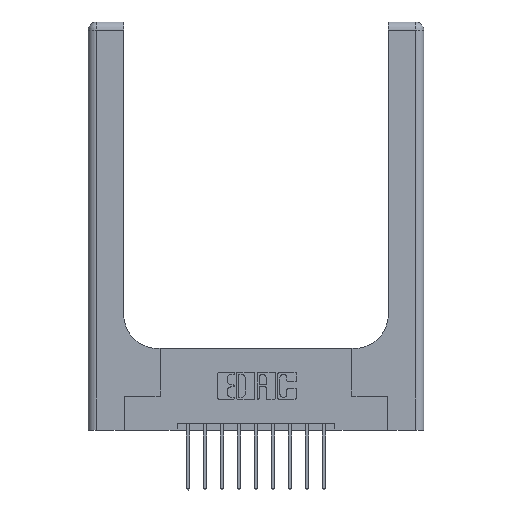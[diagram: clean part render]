
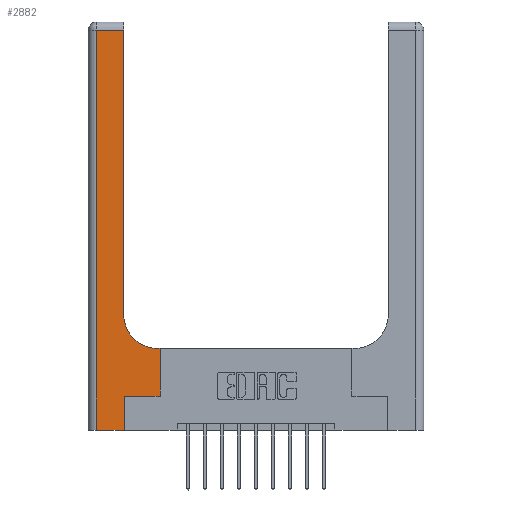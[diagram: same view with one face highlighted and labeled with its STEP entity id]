
A CAD part, top view. The second image highlights one B-rep face of the part: STEP entity #2882.
In plain terms, the highlighted planar face has unit normal (0, 0, 1).
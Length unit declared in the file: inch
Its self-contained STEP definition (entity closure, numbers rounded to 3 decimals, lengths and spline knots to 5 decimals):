
#77 = DIRECTION ( 'NONE',  ( 1., 0., 0. ) ) ;
#136 = DIRECTION ( 'NONE',  ( 0., 0., -1. ) ) ;
#170 = ORIENTED_EDGE ( 'NONE', *, *, #11150, .T. ) ;
#404 = CARTESIAN_POINT ( 'NONE',  ( 0.528, 0.6, 0.37 ) ) ;
#594 = LINE ( 'NONE', #11802, #10375 ) ;
#820 = VERTEX_POINT ( 'NONE', #9090 ) ;
#903 = LINE ( 'NONE', #4842, #3934 ) ;
#1063 = VECTOR ( 'NONE', #1886, 39.37008 ) ;
#1191 = EDGE_CURVE ( 'NONE', #10595, #3050, #9981, .T. ) ;
#1203 = CARTESIAN_POINT ( 'NONE',  ( 0., 2.94, 0.37 ) ) ;
#1225 = DIRECTION ( 'NONE',  ( 1., 0., 0. ) ) ;
#1389 = VERTEX_POINT ( 'NONE', #7661 ) ;
#1886 = DIRECTION ( 'NONE',  ( 0., 1., 0. ) ) ;
#2352 = ORIENTED_EDGE ( 'NONE', *, *, #10914, .T. ) ;
#2474 = ORIENTED_EDGE ( 'NONE', *, *, #1191, .T. ) ;
#2657 = CARTESIAN_POINT ( 'NONE',  ( 0.265, 0.25, 0.37 ) ) ;
#2847 = CARTESIAN_POINT ( 'NONE',  ( 0.528, 0.25, 0.37 ) ) ;
#2882 = ADVANCED_FACE ( 'NONE', ( #11355 ), #9747, .F. ) ;
#2932 = ORIENTED_EDGE ( 'NONE', *, *, #10328, .T. ) ;
#3050 = VERTEX_POINT ( 'NONE', #5064 ) ;
#3463 = ORIENTED_EDGE ( 'NONE', *, *, #4108, .T. ) ;
#3573 = EDGE_LOOP ( 'NONE', ( #170, #13850, #3463, #10196, #9237, #2932, #2352, #2474, #8251 ) ) ;
#3771 = DIRECTION ( 'NONE',  ( 0., -1., 0. ) ) ;
#3934 = VECTOR ( 'NONE', #13208, 39.37008 ) ;
#4108 = EDGE_CURVE ( 'NONE', #820, #1389, #4949, .T. ) ;
#4452 = LINE ( 'NONE', #10694, #8943 ) ;
#4736 = DIRECTION ( 'NONE',  ( -1., 0., 0. ) ) ;
#4842 = CARTESIAN_POINT ( 'NONE',  ( 0.265, 0.25, 0.37 ) ) ;
#4949 = LINE ( 'NONE', #8571, #5700 ) ;
#5064 = CARTESIAN_POINT ( 'NONE',  ( 0.51, 0.6, 0.37 ) ) ;
#5229 = LINE ( 'NONE', #12991, #8219 ) ;
#5380 = VERTEX_POINT ( 'NONE', #8799 ) ;
#5700 = VECTOR ( 'NONE', #3771, 39.37008 ) ;
#6095 = EDGE_CURVE ( 'NONE', #3050, #5380, #8255, .T. ) ;
#6099 = DIRECTION ( 'NONE',  ( 0., 0., -1. ) ) ;
#6612 = AXIS2_PLACEMENT_3D ( 'NONE', #13303, #136, #77 ) ;
#7354 = EDGE_CURVE ( 'NONE', #14224, #820, #14974, .T. ) ;
#7412 = VERTEX_POINT ( 'NONE', #2847 ) ;
#7661 = CARTESIAN_POINT ( 'NONE',  ( 0.06, 0., 0.37 ) ) ;
#8140 = DIRECTION ( 'NONE',  ( 0., 1., 0. ) ) ;
#8219 = VECTOR ( 'NONE', #8271, 39.37008 ) ;
#8251 = ORIENTED_EDGE ( 'NONE', *, *, #6095, .T. ) ;
#8255 = CIRCLE ( 'NONE', #6612, 0.25 ) ;
#8271 = DIRECTION ( 'NONE',  ( 0., 1., 0. ) ) ;
#8321 = EDGE_CURVE ( 'NONE', #1389, #14423, #4452, .T. ) ;
#8334 = CARTESIAN_POINT ( 'NONE',  ( 0.26, 0.6, 0.37 ) ) ;
#8426 = VERTEX_POINT ( 'NONE', #2657 ) ;
#8571 = CARTESIAN_POINT ( 'NONE',  ( 0.06, 3., 0.37 ) ) ;
#8799 = CARTESIAN_POINT ( 'NONE',  ( 0.26, 0.85, 0.37 ) ) ;
#8891 = CARTESIAN_POINT ( 'NONE',  ( 0.26, 3., 0.37 ) ) ;
#8943 = VECTOR ( 'NONE', #1225, 39.37008 ) ;
#9090 = CARTESIAN_POINT ( 'NONE',  ( 0.06, 2.94, 0.37 ) ) ;
#9163 = VECTOR ( 'NONE', #12107, 39.37008 ) ;
#9237 = ORIENTED_EDGE ( 'NONE', *, *, #14048, .T. ) ;
#9343 = LINE ( 'NONE', #8891, #1063 ) ;
#9747 = PLANE ( 'NONE',  #10409 ) ;
#9981 = LINE ( 'NONE', #8334, #11831 ) ;
#10196 = ORIENTED_EDGE ( 'NONE', *, *, #8321, .T. ) ;
#10328 = EDGE_CURVE ( 'NONE', #8426, #7412, #903, .T. ) ;
#10375 = VECTOR ( 'NONE', #8140, 39.37008 ) ;
#10409 = AXIS2_PLACEMENT_3D ( 'NONE', #11379, #6099, #13703 ) ;
#10595 = VERTEX_POINT ( 'NONE', #404 ) ;
#10694 = CARTESIAN_POINT ( 'NONE',  ( 0., 0., 0.37 ) ) ;
#10914 = EDGE_CURVE ( 'NONE', #7412, #10595, #5229, .T. ) ;
#11150 = EDGE_CURVE ( 'NONE', #5380, #14224, #9343, .T. ) ;
#11355 = FACE_OUTER_BOUND ( 'NONE', #3573, .T. ) ;
#11379 = CARTESIAN_POINT ( 'NONE',  ( 0., 3., 0.37 ) ) ;
#11802 = CARTESIAN_POINT ( 'NONE',  ( 0.265, 0., 0.37 ) ) ;
#11831 = VECTOR ( 'NONE', #4736, 39.37008 ) ;
#12107 = DIRECTION ( 'NONE',  ( -1., 0., 0. ) ) ;
#12591 = CARTESIAN_POINT ( 'NONE',  ( 0.265, 0., 0.37 ) ) ;
#12991 = CARTESIAN_POINT ( 'NONE',  ( 0.528, 0.25, 0.37 ) ) ;
#13208 = DIRECTION ( 'NONE',  ( 1., 0., 0. ) ) ;
#13303 = CARTESIAN_POINT ( 'NONE',  ( 0.51, 0.85, 0.37 ) ) ;
#13703 = DIRECTION ( 'NONE',  ( -1., 0., 0. ) ) ;
#13850 = ORIENTED_EDGE ( 'NONE', *, *, #7354, .T. ) ;
#14048 = EDGE_CURVE ( 'NONE', #14423, #8426, #594, .T. ) ;
#14224 = VERTEX_POINT ( 'NONE', #14531 ) ;
#14423 = VERTEX_POINT ( 'NONE', #12591 ) ;
#14531 = CARTESIAN_POINT ( 'NONE',  ( 0.26, 2.94, 0.37 ) ) ;
#14974 = LINE ( 'NONE', #1203, #9163 ) ;
